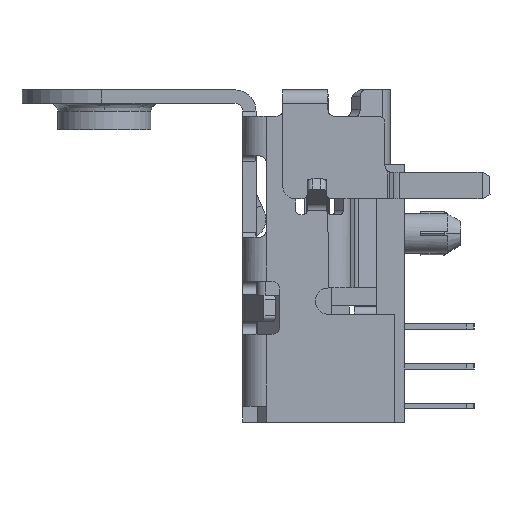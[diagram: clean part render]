
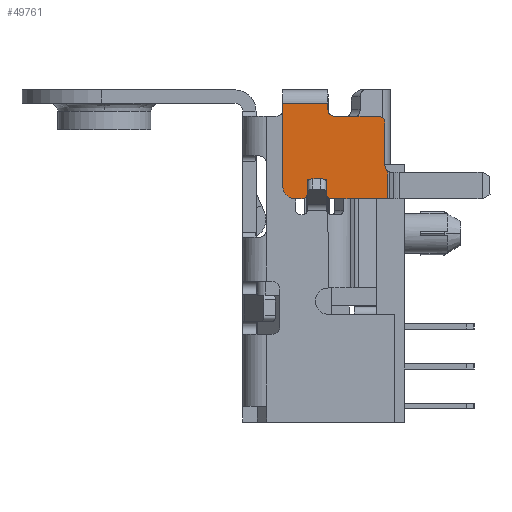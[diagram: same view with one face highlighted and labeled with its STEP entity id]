
A CAD part, left-side view. The second image highlights one B-rep face of the part: STEP entity #49761.
In plain terms, the highlighted face is planar.
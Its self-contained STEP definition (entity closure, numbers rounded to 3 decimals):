
#705 = CARTESIAN_POINT ( 'NONE',  ( 55.391, 61.575, -8.85 ) ) ;
#1395 = CIRCLE ( 'NONE', #6964, 0.25 ) ;
#1506 = VERTEX_POINT ( 'NONE', #46822 ) ;
#1555 = ORIENTED_EDGE ( 'NONE', *, *, #28384, .T. ) ;
#1793 = EDGE_CURVE ( 'NONE', #11434, #10267, #42961, .T. ) ;
#2547 = CARTESIAN_POINT ( 'NONE',  ( 55.391, 60.425, -10.65 ) ) ;
#2758 = EDGE_CURVE ( 'NONE', #10267, #44633, #52162, .T. ) ;
#3586 = VERTEX_POINT ( 'NONE', #63076 ) ;
#3697 = CARTESIAN_POINT ( 'NONE',  ( 55.391, 60.371, -12.2 ) ) ;
#3930 = ORIENTED_EDGE ( 'NONE', *, *, #11390, .T. ) ;
#4451 = ORIENTED_EDGE ( 'NONE', *, *, #45069, .T. ) ;
#4817 = EDGE_LOOP ( 'NONE', ( #46880, #24394, #36009, #24782, #39466, #59222, #67568, #4451, #44402, #40550, #26614, #18284, #50061, #23823, #3930, #1555, #8650 ) ) ;
#5395 = AXIS2_PLACEMENT_3D ( 'NONE', #46166, #62569, #14092 ) ;
#5459 = DIRECTION ( 'NONE',  ( 0., 0., 1. ) ) ;
#6226 = DIRECTION ( 'NONE',  ( 1., 0., 0. ) ) ;
#6540 = CIRCLE ( 'NONE', #5395, 0.25 ) ;
#6714 = DIRECTION ( 'NONE',  ( 0., 0., 1. ) ) ;
#6866 = DIRECTION ( 'NONE',  ( 0., 0., -1. ) ) ;
#6964 = AXIS2_PLACEMENT_3D ( 'NONE', #51844, #36465, #5459 ) ;
#8641 = VERTEX_POINT ( 'NONE', #11930 ) ;
#8650 = ORIENTED_EDGE ( 'NONE', *, *, #63373, .T. ) ;
#9713 = LINE ( 'NONE', #39806, #57646 ) ;
#9814 = DIRECTION ( 'NONE',  ( 0., 0., -1. ) ) ;
#10053 = CARTESIAN_POINT ( 'NONE',  ( 55.391, 60.1, -12.45 ) ) ;
#10130 = DIRECTION ( 'NONE',  ( -1., 0., 0. ) ) ;
#10267 = VERTEX_POINT ( 'NONE', #17070 ) ;
#10863 = DIRECTION ( 'NONE',  ( 1., 0., 0. ) ) ;
#10874 = EDGE_CURVE ( 'NONE', #41793, #23305, #43187, .T. ) ;
#11390 = EDGE_CURVE ( 'NONE', #20738, #38980, #9713, .T. ) ;
#11434 = VERTEX_POINT ( 'NONE', #51922 ) ;
#11930 = CARTESIAN_POINT ( 'NONE',  ( 55.391, 61.145, -9.56 ) ) ;
#11945 = LINE ( 'NONE', #54489, #18151 ) ;
#12021 = CARTESIAN_POINT ( 'NONE',  ( 55.391, 60.425, -9.05 ) ) ;
#12876 = AXIS2_PLACEMENT_3D ( 'NONE', #68370, #10130, #41161 ) ;
#13335 = DIRECTION ( 'NONE',  ( 0., 0., 1. ) ) ;
#14092 = DIRECTION ( 'NONE',  ( 0., 0., -1. ) ) ;
#14594 = CARTESIAN_POINT ( 'NONE',  ( 55.391, 61.145, -10.65 ) ) ;
#15269 = LINE ( 'NONE', #10053, #16894 ) ;
#16894 = VECTOR ( 'NONE', #36535, 1000. ) ;
#17070 = CARTESIAN_POINT ( 'NONE',  ( 55.391, 58.225, -10.1 ) ) ;
#17701 = EDGE_CURVE ( 'NONE', #35559, #30072, #15269, .T. ) ;
#17880 = CARTESIAN_POINT ( 'NONE',  ( 55.391, 58.125, -8.85 ) ) ;
#18023 = AXIS2_PLACEMENT_3D ( 'NONE', #25172, #10863, #9814 ) ;
#18151 = VECTOR ( 'NONE', #6714, 1000. ) ;
#18243 = EDGE_CURVE ( 'NONE', #8641, #59564, #60856, .T. ) ;
#18284 = ORIENTED_EDGE ( 'NONE', *, *, #17701, .T. ) ;
#19477 = DIRECTION ( 'NONE',  ( 0., -1., 0. ) ) ;
#19824 = DIRECTION ( 'NONE',  ( 0., 0., -1. ) ) ;
#20738 = VERTEX_POINT ( 'NONE', #705 ) ;
#20769 = CARTESIAN_POINT ( 'NONE',  ( 55.391, 58.225, -10.65 ) ) ;
#22471 = VECTOR ( 'NONE', #19477, 1000. ) ;
#23305 = VERTEX_POINT ( 'NONE', #67126 ) ;
#23588 = DIRECTION ( 'NONE',  ( 1., 0., 0. ) ) ;
#23823 = ORIENTED_EDGE ( 'NONE', *, *, #25147, .T. ) ;
#24394 = ORIENTED_EDGE ( 'NONE', *, *, #55556, .T. ) ;
#24782 = ORIENTED_EDGE ( 'NONE', *, *, #68414, .T. ) ;
#25147 = EDGE_CURVE ( 'NONE', #36508, #20738, #54618, .T. ) ;
#25172 = CARTESIAN_POINT ( 'NONE',  ( 55.391, 61.345, -9.05 ) ) ;
#26345 = CARTESIAN_POINT ( 'NONE',  ( 55.391, 60.225, -9.05 ) ) ;
#26412 = EDGE_CURVE ( 'NONE', #44282, #1506, #63069, .T. ) ;
#26614 = ORIENTED_EDGE ( 'NONE', *, *, #49724, .T. ) ;
#26985 = CARTESIAN_POINT ( 'NONE',  ( 55.391, 62.075, -9.35 ) ) ;
#26988 = CARTESIAN_POINT ( 'NONE',  ( 55.391, 58.125, -10.65 ) ) ;
#28384 = EDGE_CURVE ( 'NONE', #38980, #3586, #32512, .T. ) ;
#28682 = AXIS2_PLACEMENT_3D ( 'NONE', #26345, #32259, #68205 ) ;
#28863 = CARTESIAN_POINT ( 'NONE',  ( 55.391, 60.1, -8.85 ) ) ;
#29771 = DIRECTION ( 'NONE',  ( 0., -1., 0. ) ) ;
#30072 = VERTEX_POINT ( 'NONE', #54530 ) ;
#32259 = DIRECTION ( 'NONE',  ( 1., 0., 0. ) ) ;
#32512 = CIRCLE ( 'NONE', #18023, 0.2 ) ;
#33210 = CARTESIAN_POINT ( 'NONE',  ( 55.391, 60.371, -12.45 ) ) ;
#35559 = VERTEX_POINT ( 'NONE', #33210 ) ;
#35600 = CARTESIAN_POINT ( 'NONE',  ( 55.391, 58.225, -11.7 ) ) ;
#35866 = DIRECTION ( 'NONE',  ( 0., 0., -1. ) ) ;
#36009 = ORIENTED_EDGE ( 'NONE', *, *, #10874, .T. ) ;
#36465 = DIRECTION ( 'NONE',  ( 1., 0., 0. ) ) ;
#36508 = VERTEX_POINT ( 'NONE', #26985 ) ;
#36535 = DIRECTION ( 'NONE',  ( 0., 1., 0. ) ) ;
#36543 = LINE ( 'NONE', #67615, #51309 ) ;
#37946 = DIRECTION ( 'NONE',  ( 0., 0., 1. ) ) ;
#38283 = PLANE ( 'NONE',  #55791 ) ;
#38980 = VERTEX_POINT ( 'NONE', #67428 ) ;
#39466 = ORIENTED_EDGE ( 'NONE', *, *, #45289, .T. ) ;
#39557 = CARTESIAN_POINT ( 'NONE',  ( 55.391, 62.154, -9.56 ) ) ;
#39806 = CARTESIAN_POINT ( 'NONE',  ( 55.391, 60.1, -8.85 ) ) ;
#39997 = DIRECTION ( 'NONE',  ( 0., -1., 0. ) ) ;
#40550 = ORIENTED_EDGE ( 'NONE', *, *, #51264, .F. ) ;
#41073 = VERTEX_POINT ( 'NONE', #3697 ) ;
#41161 = DIRECTION ( 'NONE',  ( 0., 0., 1. ) ) ;
#41793 = VERTEX_POINT ( 'NONE', #12021 ) ;
#42605 = CARTESIAN_POINT ( 'NONE',  ( 55.391, 60.425, -9.56 ) ) ;
#42961 = CIRCLE ( 'NONE', #12876, 0.25 ) ;
#43035 = DIRECTION ( 'NONE',  ( 0., 0., -1. ) ) ;
#43187 = CIRCLE ( 'NONE', #28682, 0.2 ) ;
#43693 = VECTOR ( 'NONE', #29771, 1000. ) ;
#44282 = VERTEX_POINT ( 'NONE', #61280 ) ;
#44402 = ORIENTED_EDGE ( 'NONE', *, *, #26412, .F. ) ;
#44513 = CARTESIAN_POINT ( 'NONE',  ( 55.391, 61.575, -9.35 ) ) ;
#44570 = LINE ( 'NONE', #28863, #56257 ) ;
#44633 = VERTEX_POINT ( 'NONE', #35600 ) ;
#45069 = EDGE_CURVE ( 'NONE', #44633, #1506, #6540, .T. ) ;
#45289 = EDGE_CURVE ( 'NONE', #55964, #11434, #48605, .T. ) ;
#46166 = CARTESIAN_POINT ( 'NONE',  ( 55.391, 58.475, -11.7 ) ) ;
#46822 = CARTESIAN_POINT ( 'NONE',  ( 55.391, 58.475, -11.95 ) ) ;
#46880 = ORIENTED_EDGE ( 'NONE', *, *, #18243, .T. ) ;
#47931 = AXIS2_PLACEMENT_3D ( 'NONE', #44513, #23588, #6866 ) ;
#48605 = LINE ( 'NONE', #26988, #65533 ) ;
#49724 = EDGE_CURVE ( 'NONE', #41073, #35559, #36543, .T. ) ;
#49761 = ADVANCED_FACE ( 'NONE', ( #53308 ), #38283, .T. ) ;
#49873 = VECTOR ( 'NONE', #61939, 1000. ) ;
#50061 = ORIENTED_EDGE ( 'NONE', *, *, #52662, .T. ) ;
#51264 = EDGE_CURVE ( 'NONE', #41073, #44282, #1395, .T. ) ;
#51309 = VECTOR ( 'NONE', #19824, 1000. ) ;
#51844 = CARTESIAN_POINT ( 'NONE',  ( 55.391, 60.121, -12.2 ) ) ;
#51918 = CARTESIAN_POINT ( 'NONE',  ( 55.391, 59.298, -11.95 ) ) ;
#51922 = CARTESIAN_POINT ( 'NONE',  ( 55.391, 58.125, -9.9 ) ) ;
#52162 = LINE ( 'NONE', #20769, #49873 ) ;
#52662 = EDGE_CURVE ( 'NONE', #30072, #36508, #11945, .T. ) ;
#53308 = FACE_OUTER_BOUND ( 'NONE', #4817, .T. ) ;
#53599 = VECTOR ( 'NONE', #35866, 1000. ) ;
#54489 = CARTESIAN_POINT ( 'NONE',  ( 55.391, 62.075, -10.65 ) ) ;
#54530 = CARTESIAN_POINT ( 'NONE',  ( 55.391, 62.075, -12.45 ) ) ;
#54618 = CIRCLE ( 'NONE', #47931, 0.5 ) ;
#54674 = CARTESIAN_POINT ( 'NONE',  ( 55.391, 62.154, -12.522 ) ) ;
#55556 = EDGE_CURVE ( 'NONE', #59564, #41793, #61457, .T. ) ;
#55791 = AXIS2_PLACEMENT_3D ( 'NONE', #54674, #6226, #37946 ) ;
#55964 = VERTEX_POINT ( 'NONE', #17880 ) ;
#56257 = VECTOR ( 'NONE', #39997, 1000. ) ;
#56467 = LINE ( 'NONE', #14594, #53599 ) ;
#57646 = VECTOR ( 'NONE', #61102, 1000. ) ;
#59222 = ORIENTED_EDGE ( 'NONE', *, *, #1793, .T. ) ;
#59564 = VERTEX_POINT ( 'NONE', #42605 ) ;
#60856 = LINE ( 'NONE', #39557, #43693 ) ;
#61102 = DIRECTION ( 'NONE',  ( 0., -1., 0. ) ) ;
#61280 = CARTESIAN_POINT ( 'NONE',  ( 55.391, 60.121, -11.95 ) ) ;
#61457 = LINE ( 'NONE', #2547, #65251 ) ;
#61939 = DIRECTION ( 'NONE',  ( 0., 0., -1. ) ) ;
#62569 = DIRECTION ( 'NONE',  ( 1., 0., 0. ) ) ;
#63069 = LINE ( 'NONE', #51918, #22471 ) ;
#63076 = CARTESIAN_POINT ( 'NONE',  ( 55.391, 61.145, -9.05 ) ) ;
#63373 = EDGE_CURVE ( 'NONE', #3586, #8641, #56467, .T. ) ;
#65251 = VECTOR ( 'NONE', #13335, 1000. ) ;
#65533 = VECTOR ( 'NONE', #43035, 1000. ) ;
#67126 = CARTESIAN_POINT ( 'NONE',  ( 55.391, 60.225, -8.85 ) ) ;
#67428 = CARTESIAN_POINT ( 'NONE',  ( 55.391, 61.345, -8.85 ) ) ;
#67568 = ORIENTED_EDGE ( 'NONE', *, *, #2758, .T. ) ;
#67615 = CARTESIAN_POINT ( 'NONE',  ( 55.391, 60.371, -12.325 ) ) ;
#68205 = DIRECTION ( 'NONE',  ( 0., 0., -1. ) ) ;
#68370 = CARTESIAN_POINT ( 'NONE',  ( 55.391, 57.975, -10.1 ) ) ;
#68414 = EDGE_CURVE ( 'NONE', #23305, #55964, #44570, .T. ) ;
